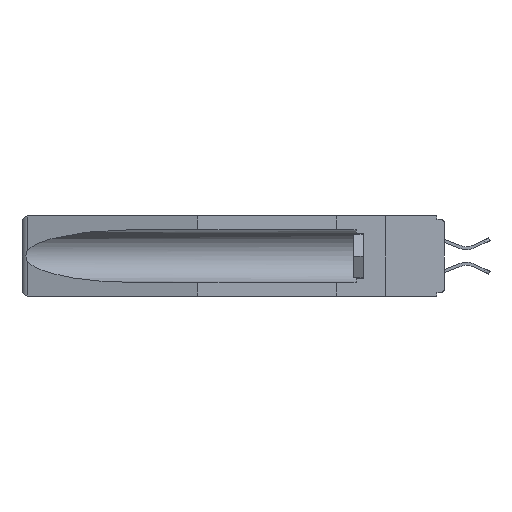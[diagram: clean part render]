
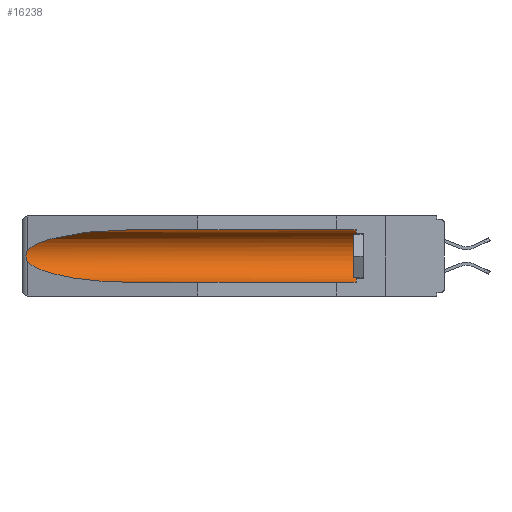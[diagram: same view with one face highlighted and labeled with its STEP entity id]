
A CAD part, left-side view. The second image highlights one B-rep face of the part: STEP entity #16238.
In plain terms, the highlighted cylindrical face has radius 2.857 mm (diameter 5.715 mm), a partial arc.
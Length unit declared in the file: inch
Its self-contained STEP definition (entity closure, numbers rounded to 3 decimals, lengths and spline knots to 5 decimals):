
#87 = EDGE_LOOP ( 'NONE', ( #8872, #27339, #1398, #12224, #23515, #7101 ) ) ;
#951 = LINE ( 'NONE', #12111, #1286 ) ;
#1239 = VERTEX_POINT ( 'NONE', #10288 ) ;
#1286 = VECTOR ( 'NONE', #20549, 39.37008 ) ;
#1398 = ORIENTED_EDGE ( 'NONE', *, *, #22084, .T. ) ;
#1800 = CARTESIAN_POINT ( 'NONE',  ( 0.26655, 1.53094, -0.18657 ) ) ;
#2135 = DIRECTION ( 'NONE',  ( 0., 1., 0. ) ) ;
#2929 = VERTEX_POINT ( 'NONE', #7407 ) ;
#3189 = EDGE_CURVE ( 'NONE', #24345, #10597, #24916, .T. ) ;
#3517 = CARTESIAN_POINT ( 'NONE',  ( 0.26537, 1.52718, -0.19328 ) ) ;
#3534 = CARTESIAN_POINT ( 'NONE',  ( 0.25451, 1.48313, -0.24835 ) ) ;
#5077 = CIRCLE ( 'NONE', #25156, 0.1125 ) ;
#5648 = CARTESIAN_POINT ( 'NONE',  ( 0.26537, 1.52718, -0.14972 ) ) ;
#5747 = CARTESIAN_POINT ( 'NONE',  ( 0.155, 1.07973, -0.284 ) ) ;
#6728 = VERTEX_POINT ( 'NONE', #3517 ) ;
#6852 = CARTESIAN_POINT ( 'NONE',  ( 0.26537, 1.52718, -0.14972 ) ) ;
#7101 = ORIENTED_EDGE ( 'NONE', *, *, #24267, .T. ) ;
#7407 = CARTESIAN_POINT ( 'NONE',  ( 0.155, 0.126, -0.059 ) ) ;
#7499 = DIRECTION ( 'NONE',  ( 0., 0., 1. ) ) ;
#8055 = CARTESIAN_POINT ( 'NONE',  ( 0.155, 0.126, -0.284 ) ) ;
#8122 = CARTESIAN_POINT ( 'NONE',  ( 0.26654, 1.53092, -0.15636 ) ) ;
#8668 = CYLINDRICAL_SURFACE ( 'NONE', #24848, 0.1125 ) ;
#8872 = ORIENTED_EDGE ( 'NONE', *, *, #13112, .T. ) ;
#9157 = CARTESIAN_POINT ( 'NONE',  ( 0.155, -0.30754, -0.1715 ) ) ;
#9468 = VECTOR ( 'NONE', #2135, 39.37008 ) ;
#9565 = CARTESIAN_POINT ( 'NONE',  ( 0.21114, 1.30732, -0.059 ) ) ;
#9636 = EDGE_CURVE ( 'NONE', #24345, #2929, #5077, .T. ) ;
#9649 = CARTESIAN_POINT ( 'NONE',  ( 0.155, 1.07973, -0.059 ) ) ;
#10288 = CARTESIAN_POINT ( 'NONE',  ( 0.155, 1.07973, -0.059 ) ) ;
#10558 = CARTESIAN_POINT ( 'NONE',  ( 0.2673, 1.53269, -0.17917 ) ) ;
#10597 = VERTEX_POINT ( 'NONE', #16648 ) ;
#10754 = VERTEX_POINT ( 'NONE', #6852 ) ;
#11985 = CARTESIAN_POINT ( 'NONE',  ( 0.21114, 1.30732, -0.284 ) ) ;
#12111 = CARTESIAN_POINT ( 'NONE',  ( 0.155, -0.30754, -0.059 ) ) ;
#12224 = ORIENTED_EDGE ( 'NONE', *, *, #3189, .F. ) ;
#13112 = EDGE_CURVE ( 'NONE', #1239, #10754, #18275, .T. ) ;
#15367 = B_SPLINE_CURVE_WITH_KNOTS ( 'NONE', 3,
 ( #5648, #20698, #8122, #25288, #23347, #25391, #10558, #1800, #23537, #27854 ),
 .UNSPECIFIED., .F., .F.,
 ( 4, 2, 2, 2, 4 ),
 ( 0., 0.00029, 0.00058, 0.00087, 0.00117 ),
 .UNSPECIFIED. ) ;
#16238 = ADVANCED_FACE ( 'NONE', ( #25086 ), #8668, .F. ) ;
#16339 = CARTESIAN_POINT ( 'NONE',  ( 0.155, 0.126, -0.1715 ) ) ;
#16557 =( BOUNDED_CURVE ( )  B_SPLINE_CURVE ( 3, ( #27019, #3534, #11985, #5747 ),
 .UNSPECIFIED., .F., .F. ) 
 B_SPLINE_CURVE_WITH_KNOTS ( ( 4, 4 ),
 ( 0.1948, 1.5708 ),
 .UNSPECIFIED. ) 
 CURVE ( )  GEOMETRIC_REPRESENTATION_ITEM ( )  RATIONAL_B_SPLINE_CURVE ( ( 1., 0.848, 0.848, 1. ) ) 
 REPRESENTATION_ITEM ( '' )  );
#16648 = CARTESIAN_POINT ( 'NONE',  ( 0.155, 1.07973, -0.284 ) ) ;
#17587 = DIRECTION ( 'NONE',  ( 0., 0., 1. ) ) ;
#18275 =( BOUNDED_CURVE ( )  B_SPLINE_CURVE ( 3, ( #9649, #9565, #22537, #24592 ),
 .UNSPECIFIED., .F., .F. ) 
 B_SPLINE_CURVE_WITH_KNOTS ( ( 4, 4 ),
 ( 4.71239, 6.08839 ),
 .UNSPECIFIED. ) 
 CURVE ( )  GEOMETRIC_REPRESENTATION_ITEM ( )  RATIONAL_B_SPLINE_CURVE ( ( 1., 0.848, 0.848, 1. ) ) 
 REPRESENTATION_ITEM ( '' )  );
#20549 = DIRECTION ( 'NONE',  ( 0., 1., 0. ) ) ;
#20562 = DIRECTION ( 'NONE',  ( 0., -1., 0. ) ) ;
#20698 = CARTESIAN_POINT ( 'NONE',  ( 0.26597, 1.52961, -0.15275 ) ) ;
#22039 = DIRECTION ( 'NONE',  ( 0., 1., 0. ) ) ;
#22084 = EDGE_CURVE ( 'NONE', #6728, #10597, #16557, .T. ) ;
#22537 = CARTESIAN_POINT ( 'NONE',  ( 0.25451, 1.48313, -0.09465 ) ) ;
#23257 = EDGE_CURVE ( 'NONE', #10754, #6728, #15367, .T. ) ;
#23347 = CARTESIAN_POINT ( 'NONE',  ( 0.2675, 1.53308, -0.16763 ) ) ;
#23515 = ORIENTED_EDGE ( 'NONE', *, *, #9636, .T. ) ;
#23537 = CARTESIAN_POINT ( 'NONE',  ( 0.26597, 1.5296, -0.19026 ) ) ;
#24267 = EDGE_CURVE ( 'NONE', #2929, #1239, #951, .T. ) ;
#24345 = VERTEX_POINT ( 'NONE', #8055 ) ;
#24592 = CARTESIAN_POINT ( 'NONE',  ( 0.26537, 1.52718, -0.14972 ) ) ;
#24848 = AXIS2_PLACEMENT_3D ( 'NONE', #9157, #22039, #17587 ) ;
#24916 = LINE ( 'NONE', #25736, #9468 ) ;
#25086 = FACE_OUTER_BOUND ( 'NONE', #87, .T. ) ;
#25156 = AXIS2_PLACEMENT_3D ( 'NONE', #16339, #20562, #7499 ) ;
#25288 = CARTESIAN_POINT ( 'NONE',  ( 0.2673, 1.5327, -0.16383 ) ) ;
#25391 = CARTESIAN_POINT ( 'NONE',  ( 0.2675, 1.53308, -0.17534 ) ) ;
#25736 = CARTESIAN_POINT ( 'NONE',  ( 0.155, -0.30754, -0.284 ) ) ;
#27019 = CARTESIAN_POINT ( 'NONE',  ( 0.26537, 1.52718, -0.19328 ) ) ;
#27339 = ORIENTED_EDGE ( 'NONE', *, *, #23257, .T. ) ;
#27854 = CARTESIAN_POINT ( 'NONE',  ( 0.26537, 1.52718, -0.19328 ) ) ;
